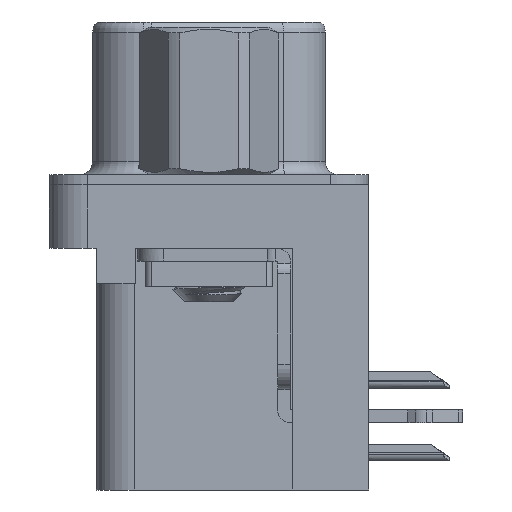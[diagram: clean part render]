
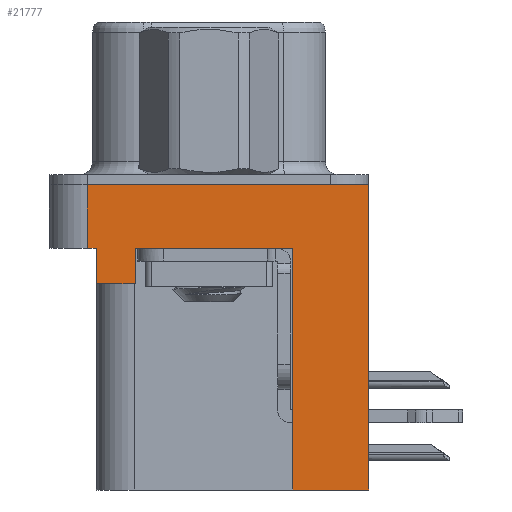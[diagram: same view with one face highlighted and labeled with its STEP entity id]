
A CAD part, left-side view. The second image highlights one B-rep face of the part: STEP entity #21777.
In plain terms, the highlighted planar face has unit normal (-1, 0, 0).
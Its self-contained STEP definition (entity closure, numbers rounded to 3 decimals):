
#574 = LINE ( 'NONE', #20630, #4672 ) ;
#603 = EDGE_CURVE ( 'NONE', #13408, #20694, #5149, .T. ) ;
#1638 = VERTEX_POINT ( 'NONE', #27312 ) ;
#2274 = ORIENTED_EDGE ( 'NONE', *, *, #13048, .F. ) ;
#2539 = DIRECTION ( 'NONE',  ( 0., 0., 1. ) ) ;
#2829 = DIRECTION ( 'NONE',  ( 0., 0., 1. ) ) ;
#2912 = EDGE_CURVE ( 'NONE', #17056, #9019, #8204, .T. ) ;
#3368 = DIRECTION ( 'NONE',  ( 0., -1., 0. ) ) ;
#3404 = EDGE_CURVE ( 'NONE', #1638, #20694, #26369, .T. ) ;
#3688 = ORIENTED_EDGE ( 'NONE', *, *, #28083, .F. ) ;
#4672 = VECTOR ( 'NONE', #22634, 1000. ) ;
#4811 = AXIS2_PLACEMENT_3D ( 'NONE', #7935, #5425, #18974 ) ;
#5149 = LINE ( 'NONE', #7253, #20976 ) ;
#5242 = EDGE_CURVE ( 'NONE', #17056, #13518, #26253, .T. ) ;
#5425 = DIRECTION ( 'NONE',  ( -1., 0., 0. ) ) ;
#5656 = LINE ( 'NONE', #14069, #22489 ) ;
#5855 = VECTOR ( 'NONE', #27367, 1000. ) ;
#6603 = ORIENTED_EDGE ( 'NONE', *, *, #5242, .T. ) ;
#7253 = CARTESIAN_POINT ( 'NONE',  ( -3., 4.425, -3.9 ) ) ;
#7750 = EDGE_CURVE ( 'NONE', #11882, #13408, #574, .T. ) ;
#7935 = CARTESIAN_POINT ( 'NONE',  ( -3., -6.275, -2.5 ) ) ;
#8204 = LINE ( 'NONE', #13745, #20909 ) ;
#8357 = DIRECTION ( 'NONE',  ( 0., -1., 0. ) ) ;
#8780 = ORIENTED_EDGE ( 'NONE', *, *, #21530, .F. ) ;
#8864 = LINE ( 'NONE', #27662, #20534 ) ;
#9019 = VERTEX_POINT ( 'NONE', #22232 ) ;
#9245 = DIRECTION ( 'NONE',  ( 0., 1., 0. ) ) ;
#9427 = DIRECTION ( 'NONE',  ( 0., 0., 1. ) ) ;
#9845 = CARTESIAN_POINT ( 'NONE',  ( -3., -6.275, 0. ) ) ;
#10169 = DIRECTION ( 'NONE',  ( 0., 0., 1. ) ) ;
#10732 = LINE ( 'NONE', #9845, #5855 ) ;
#11468 = ORIENTED_EDGE ( 'NONE', *, *, #7750, .F. ) ;
#11882 = VERTEX_POINT ( 'NONE', #25693 ) ;
#11978 = VERTEX_POINT ( 'NONE', #23311 ) ;
#13048 = EDGE_CURVE ( 'NONE', #11978, #13518, #10732, .T. ) ;
#13408 = VERTEX_POINT ( 'NONE', #26398 ) ;
#13518 = VERTEX_POINT ( 'NONE', #18135 ) ;
#13745 = CARTESIAN_POINT ( 'NONE',  ( -3., -3.295, -12. ) ) ;
#14069 = CARTESIAN_POINT ( 'NONE',  ( -3., -3.295, -12. ) ) ;
#14333 = ORIENTED_EDGE ( 'NONE', *, *, #18466, .T. ) ;
#14637 = ORIENTED_EDGE ( 'NONE', *, *, #23158, .T. ) ;
#15688 = CARTESIAN_POINT ( 'NONE',  ( -3., -6.275, -2.5 ) ) ;
#16724 = CARTESIAN_POINT ( 'NONE',  ( -3., 4.775, -2.5 ) ) ;
#17056 = VERTEX_POINT ( 'NONE', #27821 ) ;
#17446 = CARTESIAN_POINT ( 'NONE',  ( -3., 4.425, -2.5 ) ) ;
#18090 = VECTOR ( 'NONE', #10169, 1000. ) ;
#18135 = CARTESIAN_POINT ( 'NONE',  ( -3., -6.275, 0. ) ) ;
#18466 = EDGE_CURVE ( 'NONE', #11882, #19124, #24267, .T. ) ;
#18974 = DIRECTION ( 'NONE',  ( 0., 0., 1. ) ) ;
#19124 = VERTEX_POINT ( 'NONE', #21192 ) ;
#19855 = VECTOR ( 'NONE', #8357, 1000. ) ;
#19952 = LINE ( 'NONE', #16724, #23020 ) ;
#20534 = VECTOR ( 'NONE', #3368, 1000. ) ;
#20630 = CARTESIAN_POINT ( 'NONE',  ( -3., 4.425, -3.9 ) ) ;
#20694 = VERTEX_POINT ( 'NONE', #17446 ) ;
#20909 = VECTOR ( 'NONE', #9245, 1000. ) ;
#20976 = VECTOR ( 'NONE', #2539, 1000. ) ;
#21192 = CARTESIAN_POINT ( 'NONE',  ( -3., 2.895, -2.5 ) ) ;
#21466 = VECTOR ( 'NONE', #9427, 1000. ) ;
#21530 = EDGE_CURVE ( 'NONE', #1638, #11978, #19952, .T. ) ;
#21777 = ADVANCED_FACE ( 'NONE', ( #22679 ), #27708, .T. ) ;
#22232 = CARTESIAN_POINT ( 'NONE',  ( -3., -3.295, -12. ) ) ;
#22489 = VECTOR ( 'NONE', #2829, 1000. ) ;
#22634 = DIRECTION ( 'NONE',  ( 0., 1., 0. ) ) ;
#22679 = FACE_OUTER_BOUND ( 'NONE', #24071, .T. ) ;
#22780 = ORIENTED_EDGE ( 'NONE', *, *, #603, .F. ) ;
#23020 = VECTOR ( 'NONE', #25719, 1000. ) ;
#23158 = EDGE_CURVE ( 'NONE', #19124, #25787, #8864, .T. ) ;
#23311 = CARTESIAN_POINT ( 'NONE',  ( -3., 4.775, 0. ) ) ;
#24071 = EDGE_LOOP ( 'NONE', ( #2274, #8780, #27460, #22780, #11468, #14333, #14637, #3688, #24824, #6603 ) ) ;
#24267 = LINE ( 'NONE', #27959, #18090 ) ;
#24824 = ORIENTED_EDGE ( 'NONE', *, *, #2912, .F. ) ;
#25693 = CARTESIAN_POINT ( 'NONE',  ( -3., 2.895, -3.9 ) ) ;
#25717 = CARTESIAN_POINT ( 'NONE',  ( -3., -6.275, -2.5 ) ) ;
#25719 = DIRECTION ( 'NONE',  ( 0., 0., 1. ) ) ;
#25787 = VERTEX_POINT ( 'NONE', #28200 ) ;
#26253 = LINE ( 'NONE', #15688, #21466 ) ;
#26369 = LINE ( 'NONE', #25717, #19855 ) ;
#26398 = CARTESIAN_POINT ( 'NONE',  ( -3., 4.425, -3.9 ) ) ;
#27312 = CARTESIAN_POINT ( 'NONE',  ( -3., 4.775, -2.5 ) ) ;
#27367 = DIRECTION ( 'NONE',  ( 0., -1., 0. ) ) ;
#27460 = ORIENTED_EDGE ( 'NONE', *, *, #3404, .T. ) ;
#27662 = CARTESIAN_POINT ( 'NONE',  ( -3., -6.275, -2.5 ) ) ;
#27708 = PLANE ( 'NONE',  #4811 ) ;
#27821 = CARTESIAN_POINT ( 'NONE',  ( -3., -6.275, -12. ) ) ;
#27959 = CARTESIAN_POINT ( 'NONE',  ( -3., 2.895, -3.9 ) ) ;
#28083 = EDGE_CURVE ( 'NONE', #9019, #25787, #5656, .T. ) ;
#28200 = CARTESIAN_POINT ( 'NONE',  ( -3., -3.295, -2.5 ) ) ;
